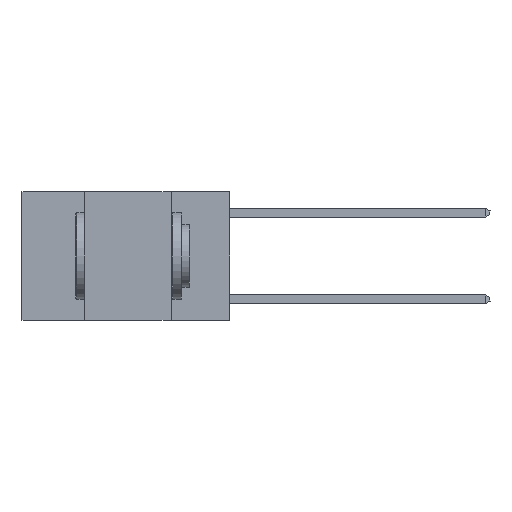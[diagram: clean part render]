
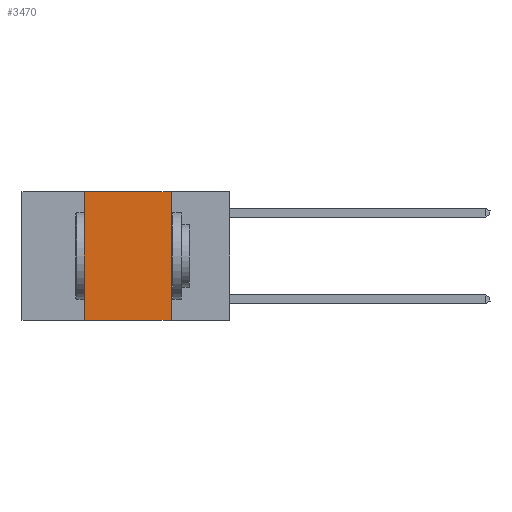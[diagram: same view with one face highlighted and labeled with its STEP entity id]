
A CAD part, left-side view. The second image highlights one B-rep face of the part: STEP entity #3470.
In plain terms, the highlighted planar face has unit normal (-1, 0, 0).
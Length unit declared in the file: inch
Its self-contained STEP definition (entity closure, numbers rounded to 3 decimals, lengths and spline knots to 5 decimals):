
#61 = VERTEX_POINT ( 'NONE', #5131 ) ;
#145 = FACE_OUTER_BOUND ( 'NONE', #3513, .T. ) ;
#789 = ORIENTED_EDGE ( 'NONE', *, *, #5521, .F. ) ;
#1541 = VERTEX_POINT ( 'NONE', #5390 ) ;
#2210 = CARTESIAN_POINT ( 'NONE',  ( 0., 0.6, -0.37 ) ) ;
#2324 = VECTOR ( 'NONE', #8696, 39.37008 ) ;
#3115 = DIRECTION ( 'NONE',  ( 0., 0., 1. ) ) ;
#3226 = EDGE_CURVE ( 'NONE', #1541, #9961, #6277, .T. ) ;
#3399 = PLANE ( 'NONE',  #4566 ) ;
#3424 = CARTESIAN_POINT ( 'NONE',  ( 0., 0.17, -0.37 ) ) ;
#3464 = VECTOR ( 'NONE', #4352, 39.37008 ) ;
#3470 = ADVANCED_FACE ( 'NONE', ( #145 ), #3399, .F. ) ;
#3513 = EDGE_LOOP ( 'NONE', ( #789, #4668, #7131, #9993 ) ) ;
#3578 = EDGE_CURVE ( 'NONE', #61, #4824, #8369, .T. ) ;
#3920 = LINE ( 'NONE', #7034, #5715 ) ;
#4123 = LINE ( 'NONE', #8939, #6133 ) ;
#4352 = DIRECTION ( 'NONE',  ( 0., -1., 0. ) ) ;
#4566 = AXIS2_PLACEMENT_3D ( 'NONE', #8264, #9878, #5055 ) ;
#4668 = ORIENTED_EDGE ( 'NONE', *, *, #3578, .F. ) ;
#4824 = VERTEX_POINT ( 'NONE', #10137 ) ;
#5055 = DIRECTION ( 'NONE',  ( 0., 0., -1. ) ) ;
#5131 = CARTESIAN_POINT ( 'NONE',  ( 0., 0.42, 0. ) ) ;
#5390 = CARTESIAN_POINT ( 'NONE',  ( 0., 0.42, -0.37 ) ) ;
#5521 = EDGE_CURVE ( 'NONE', #4824, #9961, #4123, .T. ) ;
#5715 = VECTOR ( 'NONE', #3115, 39.37008 ) ;
#6133 = VECTOR ( 'NONE', #9044, 39.37008 ) ;
#6277 = LINE ( 'NONE', #2210, #2324 ) ;
#6815 = EDGE_CURVE ( 'NONE', #1541, #61, #3920, .T. ) ;
#7034 = CARTESIAN_POINT ( 'NONE',  ( 0., 0.42, 0. ) ) ;
#7131 = ORIENTED_EDGE ( 'NONE', *, *, #6815, .F. ) ;
#7797 = CARTESIAN_POINT ( 'NONE',  ( 0., 0.6, 0. ) ) ;
#8264 = CARTESIAN_POINT ( 'NONE',  ( 0., 0.6, 0. ) ) ;
#8369 = LINE ( 'NONE', #7797, #3464 ) ;
#8696 = DIRECTION ( 'NONE',  ( 0., -1., 0. ) ) ;
#8939 = CARTESIAN_POINT ( 'NONE',  ( 0., 0.17, 0. ) ) ;
#9044 = DIRECTION ( 'NONE',  ( 0., 0., -1. ) ) ;
#9878 = DIRECTION ( 'NONE',  ( 1., 0., 0. ) ) ;
#9961 = VERTEX_POINT ( 'NONE', #3424 ) ;
#9993 = ORIENTED_EDGE ( 'NONE', *, *, #3226, .T. ) ;
#10137 = CARTESIAN_POINT ( 'NONE',  ( 0., 0.17, 0. ) ) ;
